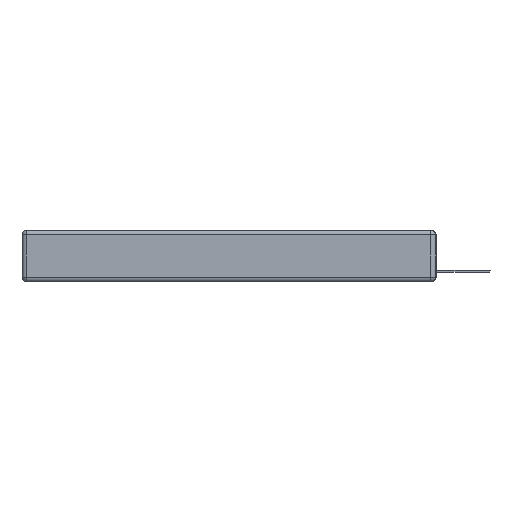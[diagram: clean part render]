
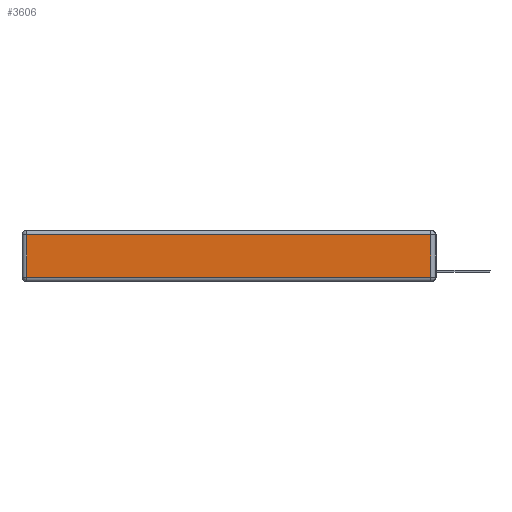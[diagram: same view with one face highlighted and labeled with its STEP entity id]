
A CAD part, left-side view. The second image highlights one B-rep face of the part: STEP entity #3606.
In plain terms, the highlighted planar face has unit normal (-1, 0, 0).
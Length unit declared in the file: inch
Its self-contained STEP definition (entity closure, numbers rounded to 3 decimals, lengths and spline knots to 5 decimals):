
#221 = EDGE_CURVE ( 'NONE', #3159, #5757, #12927, .T. ) ;
#277 = DIRECTION ( 'NONE',  ( 0., 0., 1. ) ) ;
#282 = EDGE_LOOP ( 'NONE', ( #9525, #11015, #2083, #5642 ) ) ;
#1882 = CARTESIAN_POINT ( 'NONE',  ( 0., 0.03, -0.313 ) ) ;
#2083 = ORIENTED_EDGE ( 'NONE', *, *, #16552, .T. ) ;
#3097 = VECTOR ( 'NONE', #16107, 39.37008 ) ;
#3159 = VERTEX_POINT ( 'NONE', #1882 ) ;
#3606 = ADVANCED_FACE ( 'NONE', ( #3802 ), #14344, .T. ) ;
#3802 = FACE_OUTER_BOUND ( 'NONE', #282, .T. ) ;
#4585 = VECTOR ( 'NONE', #8666, 39.37008 ) ;
#4815 = CARTESIAN_POINT ( 'NONE',  ( 0., 2.72, -0.03 ) ) ;
#5507 = LINE ( 'NONE', #10669, #3097 ) ;
#5642 = ORIENTED_EDGE ( 'NONE', *, *, #14247, .T. ) ;
#5757 = VERTEX_POINT ( 'NONE', #15264 ) ;
#6351 = EDGE_CURVE ( 'NONE', #13170, #3159, #5507, .T. ) ;
#7983 = DIRECTION ( 'NONE',  ( -1., 0., 0. ) ) ;
#8666 = DIRECTION ( 'NONE',  ( 0., 0., -1. ) ) ;
#9074 = VERTEX_POINT ( 'NONE', #4815 ) ;
#9525 = ORIENTED_EDGE ( 'NONE', *, *, #6351, .T. ) ;
#9937 = DIRECTION ( 'NONE',  ( 0., 0., 1. ) ) ;
#10053 = CARTESIAN_POINT ( 'NONE',  ( 0., 2.72, -0.343 ) ) ;
#10669 = CARTESIAN_POINT ( 'NONE',  ( 0., 0., -0.313 ) ) ;
#11015 = ORIENTED_EDGE ( 'NONE', *, *, #221, .T. ) ;
#11231 = CARTESIAN_POINT ( 'NONE',  ( 0., 0.03, -0.343 ) ) ;
#11355 = LINE ( 'NONE', #12374, #16216 ) ;
#12374 = CARTESIAN_POINT ( 'NONE',  ( 0., 2.75, -0.03 ) ) ;
#12927 = LINE ( 'NONE', #11231, #16210 ) ;
#12937 = CARTESIAN_POINT ( 'NONE',  ( 0., 2.72, -0.313 ) ) ;
#12966 = AXIS2_PLACEMENT_3D ( 'NONE', #15710, #7983, #277 ) ;
#13170 = VERTEX_POINT ( 'NONE', #12937 ) ;
#14247 = EDGE_CURVE ( 'NONE', #9074, #13170, #14462, .T. ) ;
#14344 = PLANE ( 'NONE',  #12966 ) ;
#14462 = LINE ( 'NONE', #10053, #4585 ) ;
#14915 = DIRECTION ( 'NONE',  ( 0., 1., 0. ) ) ;
#15264 = CARTESIAN_POINT ( 'NONE',  ( 0., 0.03, -0.03 ) ) ;
#15710 = CARTESIAN_POINT ( 'NONE',  ( 0., 0., -0.343 ) ) ;
#16107 = DIRECTION ( 'NONE',  ( 0., -1., 0. ) ) ;
#16210 = VECTOR ( 'NONE', #9937, 39.37008 ) ;
#16216 = VECTOR ( 'NONE', #14915, 39.37008 ) ;
#16552 = EDGE_CURVE ( 'NONE', #5757, #9074, #11355, .T. ) ;
